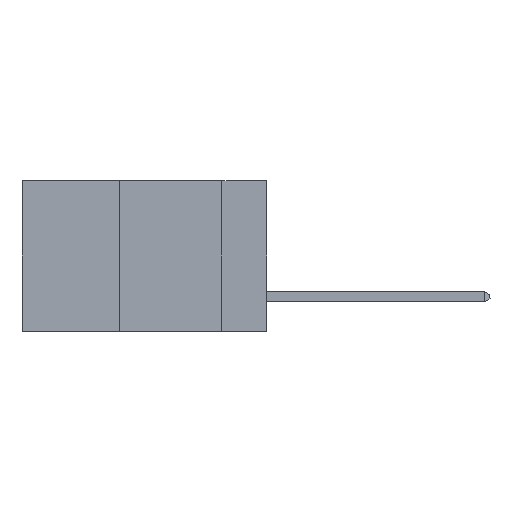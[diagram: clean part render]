
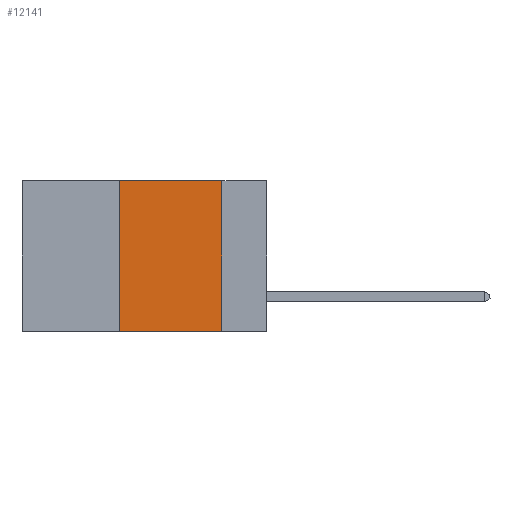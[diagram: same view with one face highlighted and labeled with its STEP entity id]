
A CAD part, left-side view. The second image highlights one B-rep face of the part: STEP entity #12141.
In plain terms, the highlighted planar face has unit normal (-1, 0, 0).
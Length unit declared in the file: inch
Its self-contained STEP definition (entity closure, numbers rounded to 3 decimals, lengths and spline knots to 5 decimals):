
#144 = FACE_OUTER_BOUND ( 'NONE', #6678, .T. ) ;
#644 = VERTEX_POINT ( 'NONE', #2804 ) ;
#665 = CARTESIAN_POINT ( 'NONE',  ( 0., 0.11, -0.37 ) ) ;
#707 = DIRECTION ( 'NONE',  ( 1., 0., 0. ) ) ;
#744 = ORIENTED_EDGE ( 'NONE', *, *, #3456, .F. ) ;
#1132 = LINE ( 'NONE', #8088, #11905 ) ;
#1420 = VERTEX_POINT ( 'NONE', #665 ) ;
#2692 = VERTEX_POINT ( 'NONE', #10544 ) ;
#2804 = CARTESIAN_POINT ( 'NONE',  ( 0., 0.36, 0. ) ) ;
#2812 = CARTESIAN_POINT ( 'NONE',  ( 0., 0.6, 0. ) ) ;
#3235 = AXIS2_PLACEMENT_3D ( 'NONE', #2812, #707, #8158 ) ;
#3456 = EDGE_CURVE ( 'NONE', #2692, #1420, #13138, .T. ) ;
#3664 = VECTOR ( 'NONE', #11179, 39.37008 ) ;
#3872 = DIRECTION ( 'NONE',  ( 0., -1., 0. ) ) ;
#4426 = ORIENTED_EDGE ( 'NONE', *, *, #13446, .T. ) ;
#4900 = VECTOR ( 'NONE', #9493, 39.37008 ) ;
#5640 = DIRECTION ( 'NONE',  ( 0., 0., -1. ) ) ;
#6585 = LINE ( 'NONE', #10165, #3664 ) ;
#6623 = CARTESIAN_POINT ( 'NONE',  ( 0., 0.36, -0.37 ) ) ;
#6678 = EDGE_LOOP ( 'NONE', ( #744, #9609, #6960, #4426 ) ) ;
#6960 = ORIENTED_EDGE ( 'NONE', *, *, #11713, .F. ) ;
#7054 = VERTEX_POINT ( 'NONE', #6623 ) ;
#7711 = LINE ( 'NONE', #12559, #4900 ) ;
#8088 = CARTESIAN_POINT ( 'NONE',  ( 0., 0.6, 0. ) ) ;
#8158 = DIRECTION ( 'NONE',  ( 0., 0., -1. ) ) ;
#9493 = DIRECTION ( 'NONE',  ( 0., 0., 1. ) ) ;
#9609 = ORIENTED_EDGE ( 'NONE', *, *, #13391, .F. ) ;
#10165 = CARTESIAN_POINT ( 'NONE',  ( 0., 0.6, -0.37 ) ) ;
#10404 = VECTOR ( 'NONE', #5640, 39.37008 ) ;
#10544 = CARTESIAN_POINT ( 'NONE',  ( 0., 0.11, 0. ) ) ;
#10664 = CARTESIAN_POINT ( 'NONE',  ( 0., 0.11, 0. ) ) ;
#11179 = DIRECTION ( 'NONE',  ( 0., -1., 0. ) ) ;
#11713 = EDGE_CURVE ( 'NONE', #7054, #644, #7711, .T. ) ;
#11905 = VECTOR ( 'NONE', #3872, 39.37008 ) ;
#12141 = ADVANCED_FACE ( 'NONE', ( #144 ), #13178, .F. ) ;
#12559 = CARTESIAN_POINT ( 'NONE',  ( 0., 0.36, 0. ) ) ;
#13138 = LINE ( 'NONE', #10664, #10404 ) ;
#13178 = PLANE ( 'NONE',  #3235 ) ;
#13391 = EDGE_CURVE ( 'NONE', #644, #2692, #1132, .T. ) ;
#13446 = EDGE_CURVE ( 'NONE', #7054, #1420, #6585, .T. ) ;
